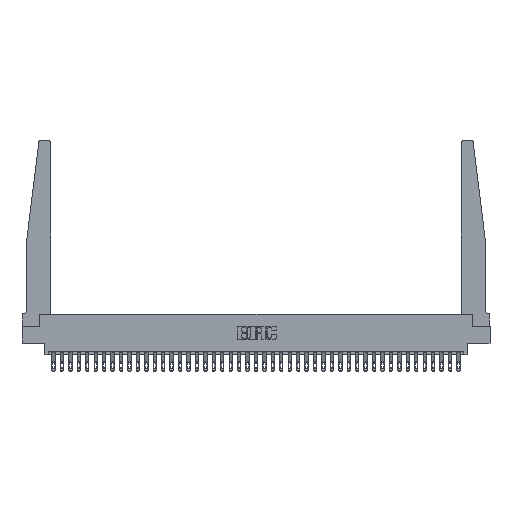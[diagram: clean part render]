
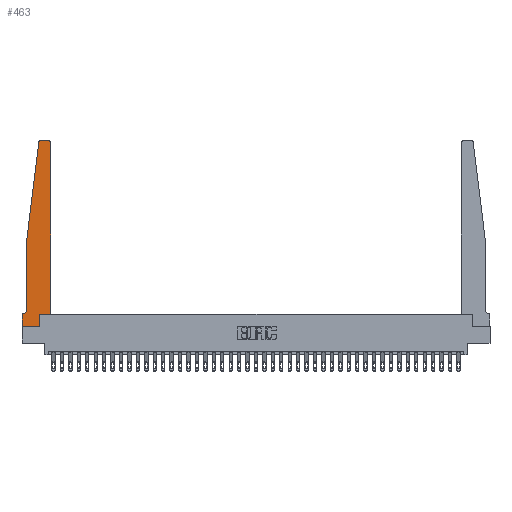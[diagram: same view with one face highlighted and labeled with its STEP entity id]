
A CAD part, top view. The second image highlights one B-rep face of the part: STEP entity #463.
In plain terms, the highlighted planar face has unit normal (0, 0, 1).
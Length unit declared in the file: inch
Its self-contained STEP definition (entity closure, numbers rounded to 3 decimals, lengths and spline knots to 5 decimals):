
#34 = CIRCLE ( 'NONE', #22391, 0.03 ) ;
#463 = ADVANCED_FACE ( 'NONE', ( #3822 ), #7894, .T. ) ;
#1193 = DIRECTION ( 'NONE',  ( 0., -1., 0. ) ) ;
#1261 = CARTESIAN_POINT ( 'NONE',  ( 0.24675, 2.72367, 0.37 ) ) ;
#1731 = ORIENTED_EDGE ( 'NONE', *, *, #17886, .T. ) ;
#2068 = CARTESIAN_POINT ( 'NONE',  ( 0., 0.1875, 0.37 ) ) ;
#2370 = LINE ( 'NONE', #29196, #31344 ) ;
#2500 = DIRECTION ( 'NONE',  ( 0., 1., 0. ) ) ;
#3093 = CIRCLE ( 'NONE', #16917, 0.03 ) ;
#3393 = CARTESIAN_POINT ( 'NONE',  ( 0.425, 2.72, 0.37 ) ) ;
#3453 = DIRECTION ( 'NONE',  ( -1., 0., 0. ) ) ;
#3567 = LINE ( 'NONE', #25438, #31658 ) ;
#3822 = FACE_OUTER_BOUND ( 'NONE', #19688, .T. ) ;
#4320 = VECTOR ( 'NONE', #32512, 39.37008 ) ;
#4388 = VECTOR ( 'NONE', #21790, 39.37008 ) ;
#4982 = CIRCLE ( 'NONE', #33334, 0.05 ) ;
#5055 = CARTESIAN_POINT ( 'NONE',  ( 0.425, 0.18, 0.37 ) ) ;
#5351 = DIRECTION ( 'NONE',  ( 1., 0., 0. ) ) ;
#5853 = DIRECTION ( 'NONE',  ( 0., 0., 1. ) ) ;
#6165 = LINE ( 'NONE', #29987, #26819 ) ;
#6804 = ORIENTED_EDGE ( 'NONE', *, *, #22108, .T. ) ;
#7146 = CARTESIAN_POINT ( 'NONE',  ( 0.27653, 2.75, 0.37 ) ) ;
#7587 = VERTEX_POINT ( 'NONE', #23043 ) ;
#7894 = PLANE ( 'NONE',  #12263 ) ;
#9590 = VERTEX_POINT ( 'NONE', #24370 ) ;
#10097 = VERTEX_POINT ( 'NONE', #7146 ) ;
#10735 = DIRECTION ( 'NONE',  ( 0., 0., 1. ) ) ;
#10782 = VECTOR ( 'NONE', #5351, 39.37008 ) ;
#10843 = ORIENTED_EDGE ( 'NONE', *, *, #31846, .T. ) ;
#11038 = CARTESIAN_POINT ( 'NONE',  ( 0.2605, 0.18, 0.37 ) ) ;
#11094 = ORIENTED_EDGE ( 'NONE', *, *, #22987, .T. ) ;
#11398 = VECTOR ( 'NONE', #3453, 39.37008 ) ;
#11482 = DIRECTION ( 'NONE',  ( -0.122, -0.992, 0. ) ) ;
#11717 = EDGE_CURVE ( 'NONE', #7587, #34253, #33079, .T. ) ;
#11916 = LINE ( 'NONE', #35646, #4388 ) ;
#12256 = CARTESIAN_POINT ( 'NONE',  ( 0.015, 0.2375, 0.37 ) ) ;
#12263 = AXIS2_PLACEMENT_3D ( 'NONE', #24707, #10735, #30307 ) ;
#12573 = VERTEX_POINT ( 'NONE', #14670 ) ;
#13165 = VERTEX_POINT ( 'NONE', #3393 ) ;
#13767 = VERTEX_POINT ( 'NONE', #28916 ) ;
#13838 = VECTOR ( 'NONE', #2500, 39.37008 ) ;
#14275 = ORIENTED_EDGE ( 'NONE', *, *, #34678, .T. ) ;
#14670 = CARTESIAN_POINT ( 'NONE',  ( 0.065, 0.2375, 0.37 ) ) ;
#14702 = CARTESIAN_POINT ( 'NONE',  ( 0.065, 0.1875, 0.37 ) ) ;
#15085 = DIRECTION ( 'NONE',  ( -1., 0., 0. ) ) ;
#15105 = CARTESIAN_POINT ( 'NONE',  ( 0.015, 0.1875, 0.37 ) ) ;
#15552 = DIRECTION ( 'NONE',  ( 0., 0., 1. ) ) ;
#15944 = CARTESIAN_POINT ( 'NONE',  ( 0.065, 1.25, 0.37 ) ) ;
#15966 = EDGE_CURVE ( 'NONE', #22645, #7587, #29583, .T. ) ;
#16231 = EDGE_CURVE ( 'NONE', #12573, #24777, #4982, .T. ) ;
#16669 = ORIENTED_EDGE ( 'NONE', *, *, #23037, .T. ) ;
#16917 = AXIS2_PLACEMENT_3D ( 'NONE', #32268, #15552, #35027 ) ;
#17244 = VECTOR ( 'NONE', #32775, 39.37008 ) ;
#17886 = EDGE_CURVE ( 'NONE', #10097, #30282, #34, .T. ) ;
#18760 = ORIENTED_EDGE ( 'NONE', *, *, #20076, .T. ) ;
#18854 = LINE ( 'NONE', #14702, #11398 ) ;
#19308 = CARTESIAN_POINT ( 'NONE',  ( 0.395, 2.75, 0.37 ) ) ;
#19688 = EDGE_LOOP ( 'NONE', ( #11094, #1731, #6804, #10843, #24908, #14275, #23279, #18760, #31036, #20351, #16669, #23467 ) ) ;
#20076 = EDGE_CURVE ( 'NONE', #13767, #22645, #34104, .T. ) ;
#20341 = CARTESIAN_POINT ( 'NONE',  ( 0.2605, 0., 0.37 ) ) ;
#20351 = ORIENTED_EDGE ( 'NONE', *, *, #11717, .T. ) ;
#21790 = DIRECTION ( 'NONE',  ( 0., 1., 0. ) ) ;
#22108 = EDGE_CURVE ( 'NONE', #30282, #9590, #3567, .T. ) ;
#22391 = AXIS2_PLACEMENT_3D ( 'NONE', #22682, #5853, #25507 ) ;
#22645 = VERTEX_POINT ( 'NONE', #20341 ) ;
#22682 = CARTESIAN_POINT ( 'NONE',  ( 0.27653, 2.72, 0.37 ) ) ;
#22987 = EDGE_CURVE ( 'NONE', #34331, #10097, #6165, .T. ) ;
#23037 = EDGE_CURVE ( 'NONE', #34253, #13165, #11916, .T. ) ;
#23043 = CARTESIAN_POINT ( 'NONE',  ( 0.2605, 0.18, 0.37 ) ) ;
#23279 = ORIENTED_EDGE ( 'NONE', *, *, #27006, .T. ) ;
#23467 = ORIENTED_EDGE ( 'NONE', *, *, #32388, .T. ) ;
#24230 = CARTESIAN_POINT ( 'NONE',  ( 0., 0., 0.37 ) ) ;
#24370 = CARTESIAN_POINT ( 'NONE',  ( 0.065, 1.25, 0.37 ) ) ;
#24383 = DIRECTION ( 'NONE',  ( -1., 0., 0. ) ) ;
#24701 = LINE ( 'NONE', #15944, #17244 ) ;
#24707 = CARTESIAN_POINT ( 'NONE',  ( 0., 0.1875, 0.37 ) ) ;
#24777 = VERTEX_POINT ( 'NONE', #15105 ) ;
#24908 = ORIENTED_EDGE ( 'NONE', *, *, #16231, .T. ) ;
#25438 = CARTESIAN_POINT ( 'NONE',  ( 0.065, 1.25, 0.37 ) ) ;
#25507 = DIRECTION ( 'NONE',  ( 1., 0., 0. ) ) ;
#26819 = VECTOR ( 'NONE', #24383, 39.37008 ) ;
#27006 = EDGE_CURVE ( 'NONE', #32545, #13767, #2370, .T. ) ;
#27675 = CARTESIAN_POINT ( 'NONE',  ( 0.425, 0.18, 0.37 ) ) ;
#28916 = CARTESIAN_POINT ( 'NONE',  ( 0., 0., 0.37 ) ) ;
#29196 = CARTESIAN_POINT ( 'NONE',  ( 0., 0., 0.37 ) ) ;
#29583 = LINE ( 'NONE', #11038, #13838 ) ;
#29987 = CARTESIAN_POINT ( 'NONE',  ( 0.25, 2.75, 0.37 ) ) ;
#30282 = VERTEX_POINT ( 'NONE', #1261 ) ;
#30307 = DIRECTION ( 'NONE',  ( 1., 0., 0. ) ) ;
#31036 = ORIENTED_EDGE ( 'NONE', *, *, #15966, .T. ) ;
#31344 = VECTOR ( 'NONE', #1193, 39.37008 ) ;
#31658 = VECTOR ( 'NONE', #11482, 39.37008 ) ;
#31805 = DIRECTION ( 'NONE',  ( 0., 0., -1. ) ) ;
#31846 = EDGE_CURVE ( 'NONE', #9590, #12573, #24701, .T. ) ;
#32268 = CARTESIAN_POINT ( 'NONE',  ( 0.395, 2.72, 0.37 ) ) ;
#32388 = EDGE_CURVE ( 'NONE', #13165, #34331, #3093, .T. ) ;
#32512 = DIRECTION ( 'NONE',  ( 1., 0., 0. ) ) ;
#32545 = VERTEX_POINT ( 'NONE', #2068 ) ;
#32775 = DIRECTION ( 'NONE',  ( 0., -1., 0. ) ) ;
#33079 = LINE ( 'NONE', #27675, #10782 ) ;
#33334 = AXIS2_PLACEMENT_3D ( 'NONE', #12256, #31805, #15085 ) ;
#34104 = LINE ( 'NONE', #24230, #4320 ) ;
#34253 = VERTEX_POINT ( 'NONE', #5055 ) ;
#34331 = VERTEX_POINT ( 'NONE', #19308 ) ;
#34678 = EDGE_CURVE ( 'NONE', #24777, #32545, #18854, .T. ) ;
#35027 = DIRECTION ( 'NONE',  ( 1., 0., 0. ) ) ;
#35646 = CARTESIAN_POINT ( 'NONE',  ( 0.425, 0.18, 0.37 ) ) ;
